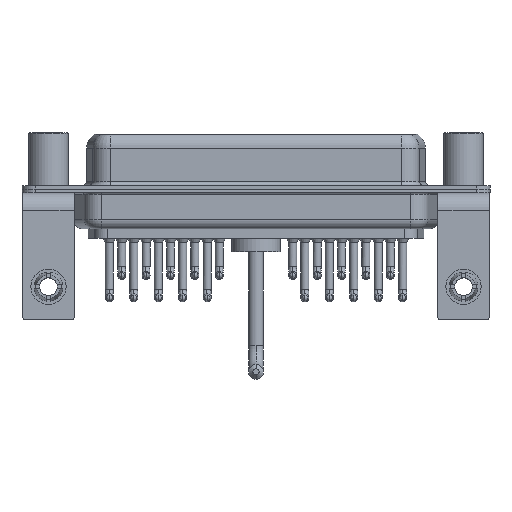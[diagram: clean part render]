
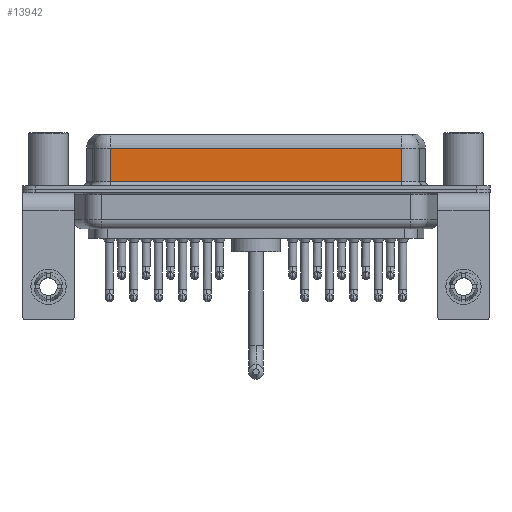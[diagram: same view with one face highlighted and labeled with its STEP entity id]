
A CAD part, front view. The second image highlights one B-rep face of the part: STEP entity #13942.
In plain terms, the highlighted planar face has unit normal (0, -1, 0).
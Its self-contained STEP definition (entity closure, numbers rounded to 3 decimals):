
#445 = CARTESIAN_POINT ( 'NONE',  ( 7.013, -3.95, 6.4 ) ) ;
#549 = ORIENTED_EDGE ( 'NONE', *, *, #20917, .F. ) ;
#1376 = CARTESIAN_POINT ( 'NONE',  ( 7.013, -3.95, 0.9 ) ) ;
#1483 = ORIENTED_EDGE ( 'NONE', *, *, #21859, .T. ) ;
#1578 = EDGE_LOOP ( 'NONE', ( #549, #14100, #6812, #1483 ) ) ;
#2718 = DIRECTION ( 'NONE',  ( 0., 0., -1. ) ) ;
#3587 = VERTEX_POINT ( 'NONE', #15292 ) ;
#4375 = DIRECTION ( 'NONE',  ( -1., 0., 0. ) ) ;
#6342 = LINE ( 'NONE', #22519, #20345 ) ;
#6812 = ORIENTED_EDGE ( 'NONE', *, *, #7376, .T. ) ;
#6851 = DIRECTION ( 'NONE',  ( 0., 0., -1. ) ) ;
#7376 = EDGE_CURVE ( 'NONE', #3587, #19242, #18582, .T. ) ;
#11370 = EDGE_CURVE ( 'NONE', #20189, #3587, #6342, .T. ) ;
#11742 = VECTOR ( 'NONE', #19048, 1000. ) ;
#12478 = PLANE ( 'NONE',  #14918 ) ;
#12745 = DIRECTION ( 'NONE',  ( 0., 0., 1. ) ) ;
#13942 = ADVANCED_FACE ( 'NONE', ( #16480 ), #12478, .F. ) ;
#13960 = CARTESIAN_POINT ( 'NONE',  ( 40.037, -3.95, 4.65 ) ) ;
#14100 = ORIENTED_EDGE ( 'NONE', *, *, #11370, .T. ) ;
#14484 = CARTESIAN_POINT ( 'NONE',  ( 40.037, -3.95, 6.4 ) ) ;
#14918 = AXIS2_PLACEMENT_3D ( 'NONE', #14484, #18856, #12745 ) ;
#14941 = CARTESIAN_POINT ( 'NONE',  ( 40.037, -3.95, 0.9 ) ) ;
#15292 = CARTESIAN_POINT ( 'NONE',  ( 7.013, -3.95, 4.65 ) ) ;
#16375 = VECTOR ( 'NONE', #6851, 1000. ) ;
#16480 = FACE_OUTER_BOUND ( 'NONE', #1578, .T. ) ;
#16732 = VERTEX_POINT ( 'NONE', #25185 ) ;
#16937 = LINE ( 'NONE', #17199, #16375 ) ;
#17199 = CARTESIAN_POINT ( 'NONE',  ( 40.037, -3.95, 6.4 ) ) ;
#18582 = LINE ( 'NONE', #445, #21937 ) ;
#18856 = DIRECTION ( 'NONE',  ( 0., 1., 0. ) ) ;
#19048 = DIRECTION ( 'NONE',  ( 1., 0., 0. ) ) ;
#19242 = VERTEX_POINT ( 'NONE', #1376 ) ;
#20189 = VERTEX_POINT ( 'NONE', #13960 ) ;
#20345 = VECTOR ( 'NONE', #4375, 1000. ) ;
#20905 = LINE ( 'NONE', #14941, #11742 ) ;
#20917 = EDGE_CURVE ( 'NONE', #20189, #16732, #16937, .T. ) ;
#21859 = EDGE_CURVE ( 'NONE', #19242, #16732, #20905, .T. ) ;
#21937 = VECTOR ( 'NONE', #2718, 1000. ) ;
#22519 = CARTESIAN_POINT ( 'NONE',  ( 40.037, -3.95, 4.65 ) ) ;
#25185 = CARTESIAN_POINT ( 'NONE',  ( 40.037, -3.95, 0.9 ) ) ;
